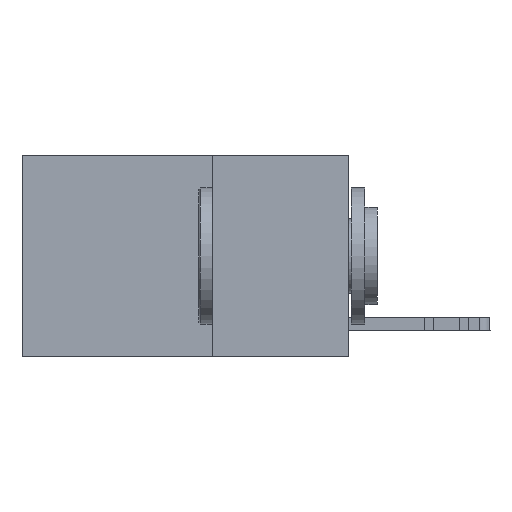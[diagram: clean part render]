
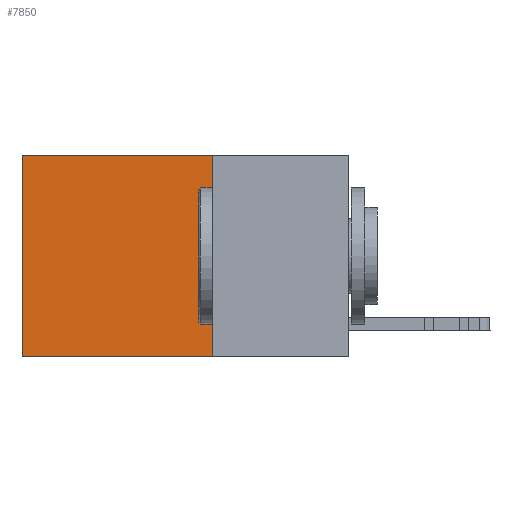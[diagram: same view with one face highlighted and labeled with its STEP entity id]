
A CAD part, left-side view. The second image highlights one B-rep face of the part: STEP entity #7850.
In plain terms, the highlighted planar face has unit normal (-1, 0, 0).
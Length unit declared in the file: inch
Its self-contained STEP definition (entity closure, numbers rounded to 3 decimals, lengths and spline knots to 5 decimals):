
#65 = VERTEX_POINT ( 'NONE', #12193 ) ;
#116 = PLANE ( 'NONE',  #15599 ) ;
#999 = CARTESIAN_POINT ( 'NONE',  ( 0.2625, 0.6, 0. ) ) ;
#2304 = FACE_OUTER_BOUND ( 'NONE', #3646, .T. ) ;
#2984 = EDGE_CURVE ( 'NONE', #18833, #22867, #6811, .T. ) ;
#3497 = LINE ( 'NONE', #12470, #15406 ) ;
#3646 = EDGE_LOOP ( 'NONE', ( #29026, #12774, #4390, #15139 ) ) ;
#3693 = EDGE_CURVE ( 'NONE', #18833, #26183, #3497, .T. ) ;
#4390 = ORIENTED_EDGE ( 'NONE', *, *, #3693, .F. ) ;
#6811 = LINE ( 'NONE', #24744, #13804 ) ;
#7850 = ADVANCED_FACE ( 'NONE', ( #2304 ), #116, .F. ) ;
#8551 = CARTESIAN_POINT ( 'NONE',  ( 0.2625, 0.25, 0. ) ) ;
#12193 = CARTESIAN_POINT ( 'NONE',  ( 0.2625, 0.6, -0.37 ) ) ;
#12470 = CARTESIAN_POINT ( 'NONE',  ( 0.2625, 0.25, 0. ) ) ;
#12774 = ORIENTED_EDGE ( 'NONE', *, *, #28878, .F. ) ;
#13004 = CARTESIAN_POINT ( 'NONE',  ( 0.2625, 0.6, 0. ) ) ;
#13804 = VECTOR ( 'NONE', #24295, 39.37008 ) ;
#14467 = VECTOR ( 'NONE', #25533, 39.37008 ) ;
#14652 = LINE ( 'NONE', #999, #14467 ) ;
#15139 = ORIENTED_EDGE ( 'NONE', *, *, #2984, .T. ) ;
#15406 = VECTOR ( 'NONE', #17019, 39.37008 ) ;
#15599 = AXIS2_PLACEMENT_3D ( 'NONE', #18011, #24948, #18150 ) ;
#17019 = DIRECTION ( 'NONE',  ( 0., 0., -1. ) ) ;
#17999 = CARTESIAN_POINT ( 'NONE',  ( 0.2625, 0.25, -0.37 ) ) ;
#18011 = CARTESIAN_POINT ( 'NONE',  ( 0.2625, 0.25, 0. ) ) ;
#18150 = DIRECTION ( 'NONE',  ( 0., 0., -1. ) ) ;
#18393 = LINE ( 'NONE', #24892, #20147 ) ;
#18833 = VERTEX_POINT ( 'NONE', #8551 ) ;
#20147 = VECTOR ( 'NONE', #21969, 39.37008 ) ;
#21969 = DIRECTION ( 'NONE',  ( 0., 1., 0. ) ) ;
#22867 = VERTEX_POINT ( 'NONE', #13004 ) ;
#24295 = DIRECTION ( 'NONE',  ( 0., 1., 0. ) ) ;
#24744 = CARTESIAN_POINT ( 'NONE',  ( 0.2625, 0.25, 0. ) ) ;
#24892 = CARTESIAN_POINT ( 'NONE',  ( 0.2625, 0.25, -0.37 ) ) ;
#24948 = DIRECTION ( 'NONE',  ( 1., 0., 0. ) ) ;
#25533 = DIRECTION ( 'NONE',  ( 0., 0., -1. ) ) ;
#26183 = VERTEX_POINT ( 'NONE', #17999 ) ;
#27130 = EDGE_CURVE ( 'NONE', #22867, #65, #14652, .T. ) ;
#28878 = EDGE_CURVE ( 'NONE', #26183, #65, #18393, .T. ) ;
#29026 = ORIENTED_EDGE ( 'NONE', *, *, #27130, .T. ) ;
